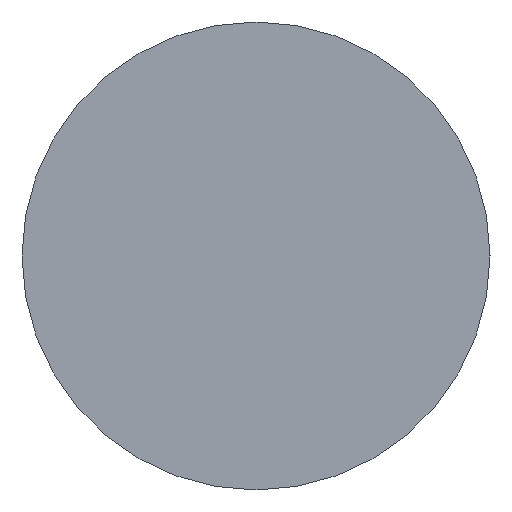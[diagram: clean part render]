
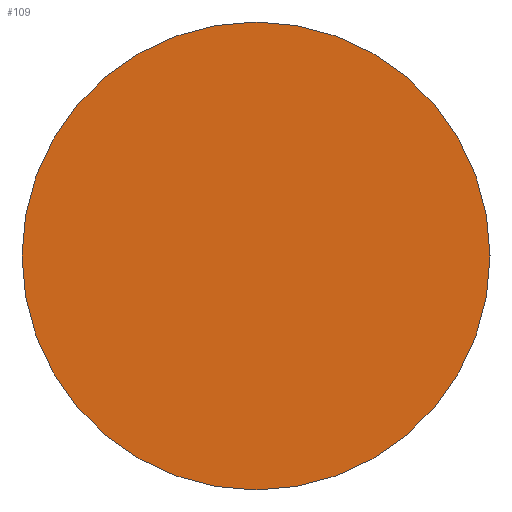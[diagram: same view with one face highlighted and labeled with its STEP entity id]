
A CAD part, left-side view. The second image highlights one B-rep face of the part: STEP entity #109.
In plain terms, the highlighted planar face has unit normal (-1, 0, 0).
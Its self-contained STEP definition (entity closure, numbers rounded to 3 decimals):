
#1 = CARTESIAN_POINT ( 'NONE',  ( 0., 0., 0. ) ) ;
#59 = AXIS2_PLACEMENT_3D ( 'NONE', #1, #150, #149 ) ;
#60 = DIRECTION ( 'NONE',  ( 1., 0., 0. ) ) ;
#62 = AXIS2_PLACEMENT_3D ( 'NONE', #159, #158, #155 ) ;
#63 = DIRECTION ( 'NONE',  ( 0., 0., -1. ) ) ;
#67 = CARTESIAN_POINT ( 'NONE',  ( 0., 0., 0. ) ) ;
#69 = CARTESIAN_POINT ( 'NONE',  ( 0., 0., 5. ) ) ;
#71 = CARTESIAN_POINT ( 'NONE',  ( 0., 0., -5. ) ) ;
#72 = AXIS2_PLACEMENT_3D ( 'NONE', #67, #60, #63 ) ;
#75 = EDGE_CURVE ( 'NONE', #171, #172, #166, .T. ) ;
#86 = EDGE_CURVE ( 'NONE', #172, #171, #139, .T. ) ;
#109 = ADVANCED_FACE ( 'NONE', ( #143 ), #162, .F. ) ;
#139 = CIRCLE ( 'NONE', #62, 5. ) ;
#143 = FACE_OUTER_BOUND ( 'NONE', #174, .T. ) ;
#149 = DIRECTION ( 'NONE',  ( 0., 0., -1. ) ) ;
#150 = DIRECTION ( 'NONE',  ( 1., 0., 0. ) ) ;
#155 = DIRECTION ( 'NONE',  ( 0., 0., -1. ) ) ;
#158 = DIRECTION ( 'NONE',  ( 1., 0., 0. ) ) ;
#159 = CARTESIAN_POINT ( 'NONE',  ( 0., 0., 0. ) ) ;
#162 = PLANE ( 'NONE',  #59 ) ;
#166 = CIRCLE ( 'NONE', #72, 5. ) ;
#168 = ORIENTED_EDGE ( 'NONE', *, *, #86, .F. ) ;
#170 = ORIENTED_EDGE ( 'NONE', *, *, #75, .F. ) ;
#171 = VERTEX_POINT ( 'NONE', #71 ) ;
#172 = VERTEX_POINT ( 'NONE', #69 ) ;
#174 = EDGE_LOOP ( 'NONE', ( #168, #170 ) ) ;
